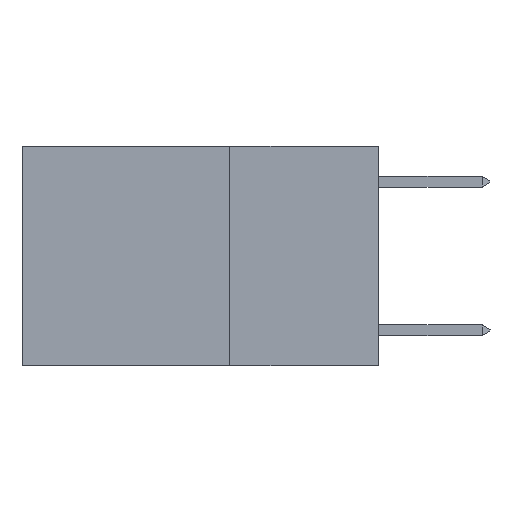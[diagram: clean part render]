
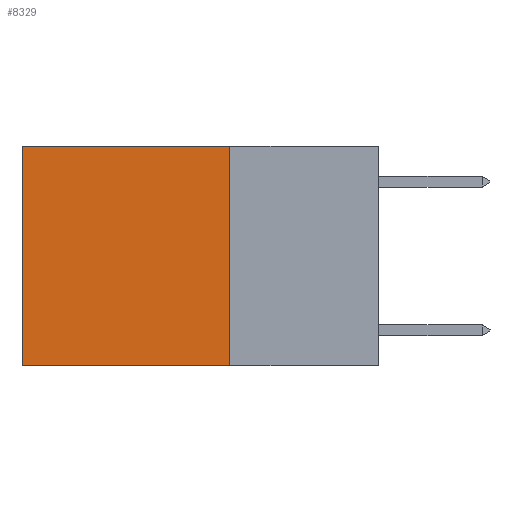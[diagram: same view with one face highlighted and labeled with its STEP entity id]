
A CAD part, left-side view. The second image highlights one B-rep face of the part: STEP entity #8329.
In plain terms, the highlighted planar face has unit normal (-1, 0, 0).
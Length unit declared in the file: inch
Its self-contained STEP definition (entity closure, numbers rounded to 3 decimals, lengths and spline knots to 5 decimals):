
#589 = DIRECTION ( 'NONE',  ( 0., 0., -1. ) ) ;
#751 = LINE ( 'NONE', #15202, #13353 ) ;
#1584 = EDGE_CURVE ( 'NONE', #5185, #1852, #3379, .T. ) ;
#1852 = VERTEX_POINT ( 'NONE', #12375 ) ;
#2720 = CARTESIAN_POINT ( 'NONE',  ( 0.2625, 0.25, -0.37 ) ) ;
#3322 = ORIENTED_EDGE ( 'NONE', *, *, #8134, .F. ) ;
#3379 = LINE ( 'NONE', #10606, #15559 ) ;
#3932 = AXIS2_PLACEMENT_3D ( 'NONE', #13613, #6315, #14842 ) ;
#4927 = FACE_OUTER_BOUND ( 'NONE', #15162, .T. ) ;
#5185 = VERTEX_POINT ( 'NONE', #8256 ) ;
#5959 = CARTESIAN_POINT ( 'NONE',  ( 0.2625, 0.25, 0. ) ) ;
#6315 = DIRECTION ( 'NONE',  ( 1., 0., 0. ) ) ;
#6658 = EDGE_CURVE ( 'NONE', #1852, #15317, #751, .T. ) ;
#6859 = ORIENTED_EDGE ( 'NONE', *, *, #1584, .T. ) ;
#7200 = VERTEX_POINT ( 'NONE', #2720 ) ;
#7941 = LINE ( 'NONE', #5959, #14074 ) ;
#7977 = ORIENTED_EDGE ( 'NONE', *, *, #13525, .F. ) ;
#8134 = EDGE_CURVE ( 'NONE', #5185, #7200, #7941, .T. ) ;
#8256 = CARTESIAN_POINT ( 'NONE',  ( 0.2625, 0.25, 0. ) ) ;
#8329 = ADVANCED_FACE ( 'NONE', ( #4927 ), #11146, .F. ) ;
#10271 = CARTESIAN_POINT ( 'NONE',  ( 0.2625, 0.6, -0.37 ) ) ;
#10606 = CARTESIAN_POINT ( 'NONE',  ( 0.2625, 0.25, 0. ) ) ;
#11146 = PLANE ( 'NONE',  #3932 ) ;
#11386 = ORIENTED_EDGE ( 'NONE', *, *, #6658, .T. ) ;
#11513 = DIRECTION ( 'NONE',  ( 0., 1., 0. ) ) ;
#12375 = CARTESIAN_POINT ( 'NONE',  ( 0.2625, 0.6, 0. ) ) ;
#12702 = CARTESIAN_POINT ( 'NONE',  ( 0.2625, 0.25, -0.37 ) ) ;
#13102 = DIRECTION ( 'NONE',  ( 0., 1., 0. ) ) ;
#13353 = VECTOR ( 'NONE', #589, 39.37008 ) ;
#13525 = EDGE_CURVE ( 'NONE', #7200, #15317, #14363, .T. ) ;
#13597 = VECTOR ( 'NONE', #11513, 39.37008 ) ;
#13613 = CARTESIAN_POINT ( 'NONE',  ( 0.2625, 0.25, 0. ) ) ;
#14074 = VECTOR ( 'NONE', #14484, 39.37008 ) ;
#14363 = LINE ( 'NONE', #12702, #13597 ) ;
#14484 = DIRECTION ( 'NONE',  ( 0., 0., -1. ) ) ;
#14842 = DIRECTION ( 'NONE',  ( 0., 0., -1. ) ) ;
#15162 = EDGE_LOOP ( 'NONE', ( #11386, #7977, #3322, #6859 ) ) ;
#15202 = CARTESIAN_POINT ( 'NONE',  ( 0.2625, 0.6, 0. ) ) ;
#15317 = VERTEX_POINT ( 'NONE', #10271 ) ;
#15559 = VECTOR ( 'NONE', #13102, 39.37008 ) ;
